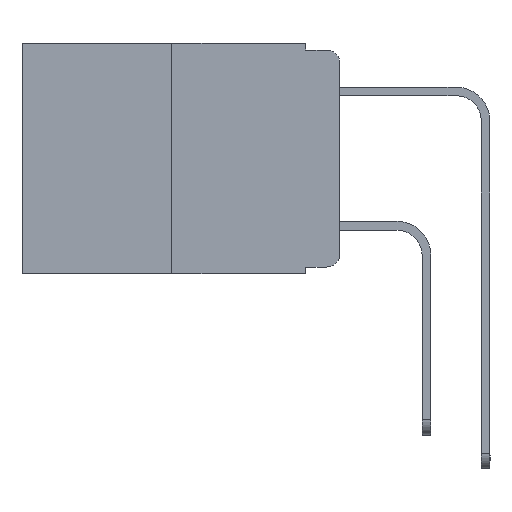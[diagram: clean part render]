
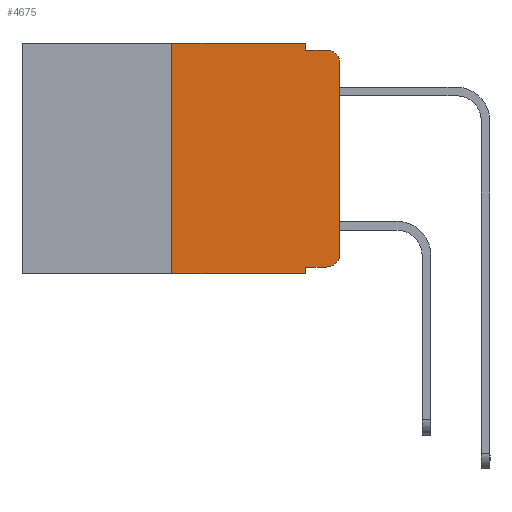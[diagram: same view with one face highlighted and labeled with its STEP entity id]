
A CAD part, left-side view. The second image highlights one B-rep face of the part: STEP entity #4675.
In plain terms, the highlighted planar face has unit normal (-1, 0, 0).
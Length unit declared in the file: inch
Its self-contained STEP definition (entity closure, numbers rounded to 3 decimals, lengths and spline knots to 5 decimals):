
#76 = VECTOR ( 'NONE', #16480, 39.37008 ) ;
#317 = EDGE_CURVE ( 'NONE', #8783, #21649, #15689, .T. ) ;
#550 = CARTESIAN_POINT ( 'NONE',  ( 0., 0.051, 0. ) ) ;
#827 = DIRECTION ( 'NONE',  ( 0., -1., 0. ) ) ;
#854 = ORIENTED_EDGE ( 'NONE', *, *, #10130, .F. ) ;
#1171 = CARTESIAN_POINT ( 'NONE',  ( 0., 0.051, 0. ) ) ;
#1422 = CARTESIAN_POINT ( 'NONE',  ( 0., 0.051, -0.01 ) ) ;
#1500 = DIRECTION ( 'NONE',  ( -1., 0., 0. ) ) ;
#1637 = ORIENTED_EDGE ( 'NONE', *, *, #2439, .T. ) ;
#1644 = CARTESIAN_POINT ( 'NONE',  ( 0., 0.02, -0.333 ) ) ;
#2023 = LINE ( 'NONE', #10110, #15530 ) ;
#2046 = LINE ( 'NONE', #16237, #10992 ) ;
#2104 = EDGE_CURVE ( 'NONE', #21318, #17237, #17730, .T. ) ;
#2130 = ORIENTED_EDGE ( 'NONE', *, *, #16603, .T. ) ;
#2439 = EDGE_CURVE ( 'NONE', #21649, #18903, #25280, .T. ) ;
#2449 = LINE ( 'NONE', #10538, #9549 ) ;
#2725 = EDGE_CURVE ( 'NONE', #6124, #23968, #2046, .T. ) ;
#3071 = CARTESIAN_POINT ( 'NONE',  ( 0., 0.473, 0. ) ) ;
#3645 = CARTESIAN_POINT ( 'NONE',  ( 0., 0.051, -0.343 ) ) ;
#3664 = CARTESIAN_POINT ( 'NONE',  ( 0., 0.02, -0.313 ) ) ;
#3798 = CARTESIAN_POINT ( 'NONE',  ( 0., 0.25, 0. ) ) ;
#3911 = VECTOR ( 'NONE', #21785, 39.37008 ) ;
#4210 = ORIENTED_EDGE ( 'NONE', *, *, #2725, .F. ) ;
#4569 = AXIS2_PLACEMENT_3D ( 'NONE', #3664, #13608, #17438 ) ;
#4675 = ADVANCED_FACE ( 'NONE', ( #15140 ), #19775, .F. ) ;
#5346 = ORIENTED_EDGE ( 'NONE', *, *, #2104, .F. ) ;
#5854 = CARTESIAN_POINT ( 'NONE',  ( 0., 0.02, -0.01 ) ) ;
#6124 = VERTEX_POINT ( 'NONE', #19956 ) ;
#6140 = DIRECTION ( 'NONE',  ( 0., -1., 0. ) ) ;
#6890 = VERTEX_POINT ( 'NONE', #16980 ) ;
#7285 = VECTOR ( 'NONE', #17969, 39.37008 ) ;
#8197 = CARTESIAN_POINT ( 'NONE',  ( 0., 0.051, -0.01 ) ) ;
#8513 = EDGE_CURVE ( 'NONE', #18903, #18834, #16695, .T. ) ;
#8572 = ORIENTED_EDGE ( 'NONE', *, *, #16795, .T. ) ;
#8783 = VERTEX_POINT ( 'NONE', #19860 ) ;
#9549 = VECTOR ( 'NONE', #18620, 39.37008 ) ;
#9786 = DIRECTION ( 'NONE',  ( 0., -1., 0. ) ) ;
#9997 = AXIS2_PLACEMENT_3D ( 'NONE', #19156, #1500, #25511 ) ;
#10110 = CARTESIAN_POINT ( 'NONE',  ( 0., 0.473, -0.343 ) ) ;
#10130 = EDGE_CURVE ( 'NONE', #6890, #6124, #14141, .T. ) ;
#10538 = CARTESIAN_POINT ( 'NONE',  ( 0., 0.051, 0. ) ) ;
#10732 = EDGE_CURVE ( 'NONE', #23968, #21318, #18737, .T. ) ;
#10992 = VECTOR ( 'NONE', #827, 39.37008 ) ;
#11158 = DIRECTION ( 'NONE',  ( 0., 0., -1. ) ) ;
#13608 = DIRECTION ( 'NONE',  ( -1., 0., 0. ) ) ;
#13853 = ORIENTED_EDGE ( 'NONE', *, *, #10732, .F. ) ;
#14141 = LINE ( 'NONE', #3798, #7285 ) ;
#14584 = DIRECTION ( 'NONE',  ( 0., 0., 1. ) ) ;
#15101 = VECTOR ( 'NONE', #9786, 39.37008 ) ;
#15140 = FACE_OUTER_BOUND ( 'NONE', #17941, .T. ) ;
#15192 = EDGE_CURVE ( 'NONE', #8783, #16753, #2449, .T. ) ;
#15530 = VECTOR ( 'NONE', #6140, 39.37008 ) ;
#15689 = LINE ( 'NONE', #23759, #3911 ) ;
#16237 = CARTESIAN_POINT ( 'NONE',  ( 0., 0.473, 0. ) ) ;
#16480 = DIRECTION ( 'NONE',  ( 0., 0., -1. ) ) ;
#16603 = EDGE_CURVE ( 'NONE', #18834, #17237, #21443, .T. ) ;
#16695 = LINE ( 'NONE', #22783, #18089 ) ;
#16753 = VERTEX_POINT ( 'NONE', #3645 ) ;
#16795 = EDGE_CURVE ( 'NONE', #6890, #16753, #2023, .T. ) ;
#16929 = AXIS2_PLACEMENT_3D ( 'NONE', #3071, #23206, #11158 ) ;
#16980 = CARTESIAN_POINT ( 'NONE',  ( 0., 0.25, -0.343 ) ) ;
#17237 = VERTEX_POINT ( 'NONE', #5854 ) ;
#17438 = DIRECTION ( 'NONE',  ( 0., 0., -1. ) ) ;
#17730 = LINE ( 'NONE', #1422, #15101 ) ;
#17941 = EDGE_LOOP ( 'NONE', ( #18936, #2130, #5346, #13853, #4210, #854, #8572, #23246, #18673, #1637 ) ) ;
#17969 = DIRECTION ( 'NONE',  ( 0., 0., 1. ) ) ;
#18089 = VECTOR ( 'NONE', #14584, 39.37008 ) ;
#18620 = DIRECTION ( 'NONE',  ( 0., 0., -1. ) ) ;
#18673 = ORIENTED_EDGE ( 'NONE', *, *, #317, .T. ) ;
#18737 = LINE ( 'NONE', #550, #76 ) ;
#18834 = VERTEX_POINT ( 'NONE', #22092 ) ;
#18903 = VERTEX_POINT ( 'NONE', #24867 ) ;
#18936 = ORIENTED_EDGE ( 'NONE', *, *, #8513, .T. ) ;
#19156 = CARTESIAN_POINT ( 'NONE',  ( 0., 0.02, -0.03 ) ) ;
#19775 = PLANE ( 'NONE',  #16929 ) ;
#19860 = CARTESIAN_POINT ( 'NONE',  ( 0., 0.051, -0.333 ) ) ;
#19956 = CARTESIAN_POINT ( 'NONE',  ( 0., 0.25, 0. ) ) ;
#21318 = VERTEX_POINT ( 'NONE', #8197 ) ;
#21443 = CIRCLE ( 'NONE', #9997, 0.02 ) ;
#21649 = VERTEX_POINT ( 'NONE', #1644 ) ;
#21785 = DIRECTION ( 'NONE',  ( 0., -1., 0. ) ) ;
#22092 = CARTESIAN_POINT ( 'NONE',  ( 0., 0., -0.03 ) ) ;
#22783 = CARTESIAN_POINT ( 'NONE',  ( 0., 0., 0. ) ) ;
#23206 = DIRECTION ( 'NONE',  ( 1., 0., 0. ) ) ;
#23246 = ORIENTED_EDGE ( 'NONE', *, *, #15192, .F. ) ;
#23759 = CARTESIAN_POINT ( 'NONE',  ( 0., 0.051, -0.333 ) ) ;
#23968 = VERTEX_POINT ( 'NONE', #1171 ) ;
#24867 = CARTESIAN_POINT ( 'NONE',  ( 0., 0., -0.313 ) ) ;
#25280 = CIRCLE ( 'NONE', #4569, 0.02 ) ;
#25511 = DIRECTION ( 'NONE',  ( 0., 0., -1. ) ) ;
